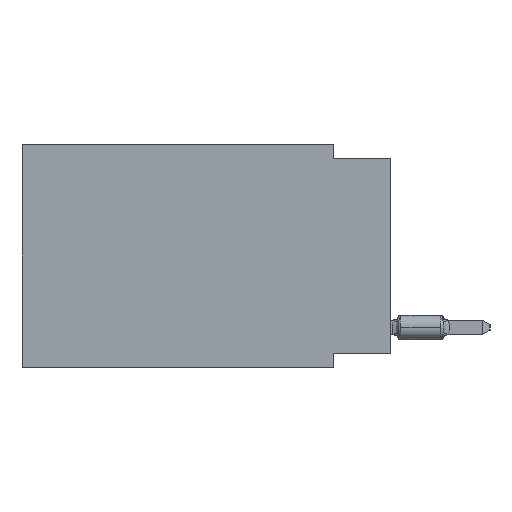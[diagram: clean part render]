
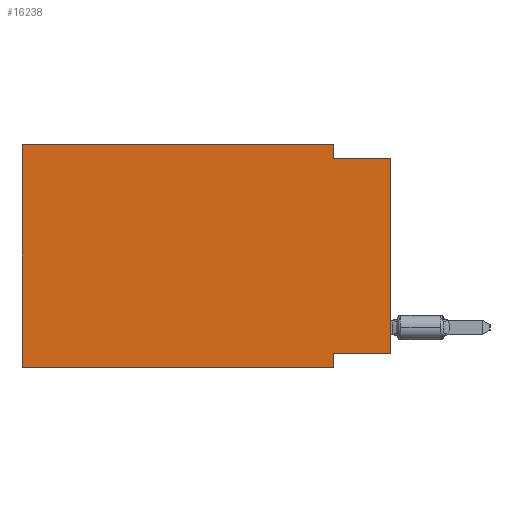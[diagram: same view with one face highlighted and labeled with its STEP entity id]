
A CAD part, left-side view. The second image highlights one B-rep face of the part: STEP entity #16238.
In plain terms, the highlighted planar face has unit normal (-1, 0, 0).
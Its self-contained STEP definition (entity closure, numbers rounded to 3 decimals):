
#752 = DIRECTION ( 'NONE',  ( 0., -1., 0. ) ) ;
#957 = LINE ( 'NONE', #26180, #4620 ) ;
#2199 = LINE ( 'NONE', #22400, #9850 ) ;
#2665 = EDGE_CURVE ( 'NONE', #16233, #18426, #28733, .T. ) ;
#2700 = LINE ( 'NONE', #22266, #9653 ) ;
#2855 = LINE ( 'NONE', #12730, #30843 ) ;
#3613 = EDGE_CURVE ( 'NONE', #19396, #18631, #19942, .T. ) ;
#3837 = VERTEX_POINT ( 'NONE', #12817 ) ;
#3861 = CARTESIAN_POINT ( 'NONE',  ( 0., 16.383, 0. ) ) ;
#4093 = ORIENTED_EDGE ( 'NONE', *, *, #6922, .F. ) ;
#4461 = ORIENTED_EDGE ( 'NONE', *, *, #6798, .F. ) ;
#4620 = VECTOR ( 'NONE', #6465, 1000. ) ;
#4631 = ORIENTED_EDGE ( 'NONE', *, *, #10517, .F. ) ;
#5554 = VERTEX_POINT ( 'NONE', #19049 ) ;
#6277 = FACE_OUTER_BOUND ( 'NONE', #6638, .T. ) ;
#6465 = DIRECTION ( 'NONE',  ( 0., 0., 1. ) ) ;
#6638 = EDGE_LOOP ( 'NONE', ( #26348, #20090, #14189, #4461, #4631, #18615, #20933, #4093 ) ) ;
#6798 = EDGE_CURVE ( 'NONE', #12778, #19396, #2700, .T. ) ;
#6922 = EDGE_CURVE ( 'NONE', #15783, #5554, #2855, .T. ) ;
#8577 = CARTESIAN_POINT ( 'NONE',  ( 0., 0., -9.271 ) ) ;
#8722 = CARTESIAN_POINT ( 'NONE',  ( 0., 2.54, 0. ) ) ;
#9023 = DIRECTION ( 'NONE',  ( 0., -1., 0. ) ) ;
#9653 = VECTOR ( 'NONE', #752, 1000. ) ;
#9722 = EDGE_CURVE ( 'NONE', #5554, #18426, #14325, .T. ) ;
#9850 = VECTOR ( 'NONE', #31799, 1000. ) ;
#10517 = EDGE_CURVE ( 'NONE', #16233, #12778, #26200, .T. ) ;
#11738 = CARTESIAN_POINT ( 'NONE',  ( 0., 2.54, -9.906 ) ) ;
#12031 = CARTESIAN_POINT ( 'NONE',  ( 0., 2.54, -0.635 ) ) ;
#12494 = VECTOR ( 'NONE', #9023, 1000. ) ;
#12730 = CARTESIAN_POINT ( 'NONE',  ( 0., 0., -9.271 ) ) ;
#12778 = VERTEX_POINT ( 'NONE', #27689 ) ;
#12817 = CARTESIAN_POINT ( 'NONE',  ( 0., 0., -0.635 ) ) ;
#14189 = ORIENTED_EDGE ( 'NONE', *, *, #3613, .F. ) ;
#14197 = DIRECTION ( 'NONE',  ( 0., 0., -1. ) ) ;
#14325 = LINE ( 'NONE', #11738, #21619 ) ;
#15783 = VERTEX_POINT ( 'NONE', #8577 ) ;
#16233 = VERTEX_POINT ( 'NONE', #18562 ) ;
#16238 = ADVANCED_FACE ( 'NONE', ( #6277 ), #26006, .F. ) ;
#18426 = VERTEX_POINT ( 'NONE', #26496 ) ;
#18562 = CARTESIAN_POINT ( 'NONE',  ( 0., 16.383, -9.906 ) ) ;
#18615 = ORIENTED_EDGE ( 'NONE', *, *, #2665, .T. ) ;
#18631 = VERTEX_POINT ( 'NONE', #12031 ) ;
#18934 = AXIS2_PLACEMENT_3D ( 'NONE', #3861, #23579, #14197 ) ;
#19049 = CARTESIAN_POINT ( 'NONE',  ( 0., 2.54, -9.271 ) ) ;
#19396 = VERTEX_POINT ( 'NONE', #8722 ) ;
#19475 = DIRECTION ( 'NONE',  ( 0., 0., -1. ) ) ;
#19942 = LINE ( 'NONE', #29957, #21845 ) ;
#20090 = ORIENTED_EDGE ( 'NONE', *, *, #20208, .F. ) ;
#20208 = EDGE_CURVE ( 'NONE', #18631, #3837, #2199, .T. ) ;
#20933 = ORIENTED_EDGE ( 'NONE', *, *, #9722, .F. ) ;
#21358 = DIRECTION ( 'NONE',  ( 0., 0., 1. ) ) ;
#21619 = VECTOR ( 'NONE', #31308, 1000. ) ;
#21845 = VECTOR ( 'NONE', #19475, 1000. ) ;
#22266 = CARTESIAN_POINT ( 'NONE',  ( 0., 16.383, 0. ) ) ;
#22400 = CARTESIAN_POINT ( 'NONE',  ( 0., 0., -0.635 ) ) ;
#22583 = DIRECTION ( 'NONE',  ( 0., 1., 0. ) ) ;
#23579 = DIRECTION ( 'NONE',  ( 1., 0., 0. ) ) ;
#23956 = CARTESIAN_POINT ( 'NONE',  ( 0., 16.383, 0. ) ) ;
#26006 = PLANE ( 'NONE',  #18934 ) ;
#26180 = CARTESIAN_POINT ( 'NONE',  ( 0., 0., 0. ) ) ;
#26200 = LINE ( 'NONE', #23956, #26272 ) ;
#26272 = VECTOR ( 'NONE', #21358, 1000. ) ;
#26348 = ORIENTED_EDGE ( 'NONE', *, *, #31216, .T. ) ;
#26496 = CARTESIAN_POINT ( 'NONE',  ( 0., 2.54, -9.906 ) ) ;
#26796 = CARTESIAN_POINT ( 'NONE',  ( 0., 16.383, -9.906 ) ) ;
#27689 = CARTESIAN_POINT ( 'NONE',  ( 0., 16.383, 0. ) ) ;
#28733 = LINE ( 'NONE', #26796, #12494 ) ;
#29957 = CARTESIAN_POINT ( 'NONE',  ( 0., 2.54, 0. ) ) ;
#30843 = VECTOR ( 'NONE', #22583, 1000. ) ;
#31216 = EDGE_CURVE ( 'NONE', #15783, #3837, #957, .T. ) ;
#31308 = DIRECTION ( 'NONE',  ( 0., 0., -1. ) ) ;
#31799 = DIRECTION ( 'NONE',  ( 0., -1., 0. ) ) ;
